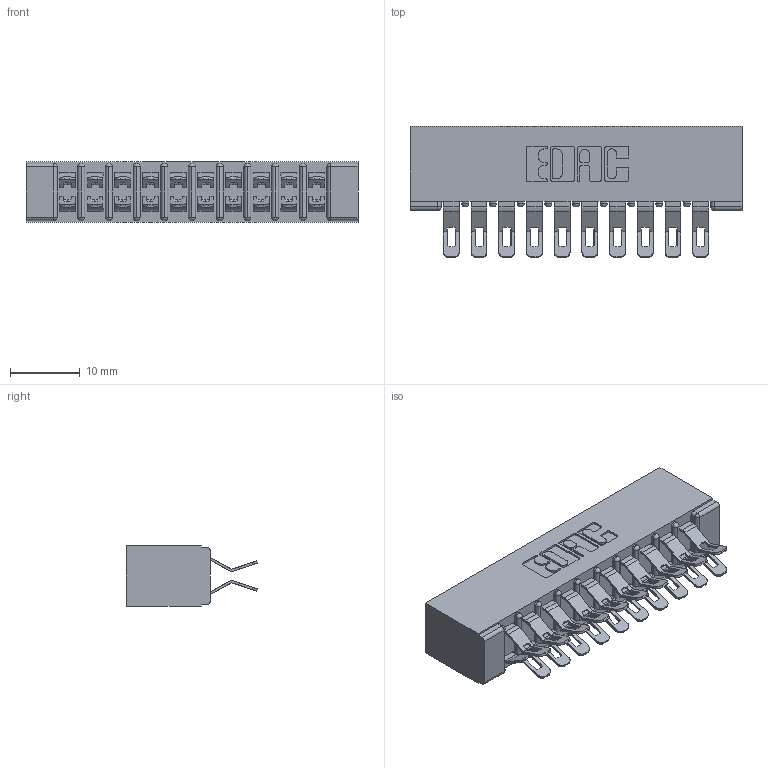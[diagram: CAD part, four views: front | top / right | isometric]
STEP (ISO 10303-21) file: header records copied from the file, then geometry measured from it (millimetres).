
FILE_DESCRIPTION (( 'STEP AP203' ), '1' );
FILE_NAME ('357-020-455-201.STEP', '2020-10-02T22:09:12', ( '' ), ( '' ), 'SwSTEP 2.0', 'SolidWorks 2020', '' );
FILE_SCHEMA (( 'CONFIG_CONTROL_DESIGN' ));
Length unit declared in the file: inch
Products named in the file (3): 357-020-455-201; 307-290-001_555; 307 Part_No Mounting Lugs
Assembly tree (21 placements, depth 2):
  357-020-455-201
    307 Part_No Mounting Lugs
    307-290-001_555  x20
Bounding box: 47.5 x 18.75 x 8.71 mm (x, y, z)
Volume: 3400.9 mm3; surface area: 6180.9 mm2
Topology: 21 solids, 21 shells, 1341 faces, 3919 edges, 2554 vertices
Faces by surface type: plane 746, cylinder 573, sphere 22
Entity records: 13097 total; most frequent: CARTESIAN_POINT 2154, ORIENTED_EDGE 2132, DIRECTION 2130, EDGE_CURVE 1066, LINE 794, VECTOR 794, VERTEX_POINT 692, AXIS2_PLACEMENT_3D 668
